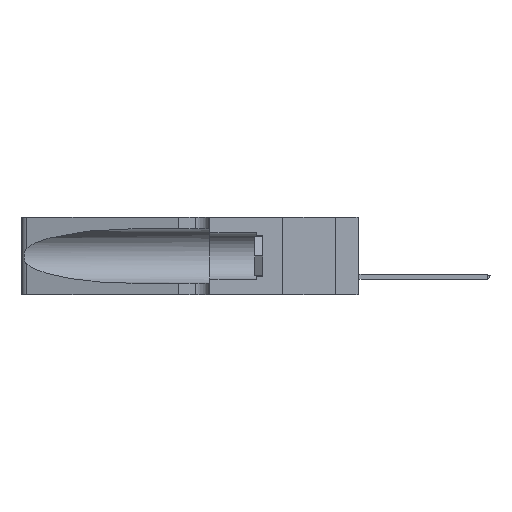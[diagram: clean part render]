
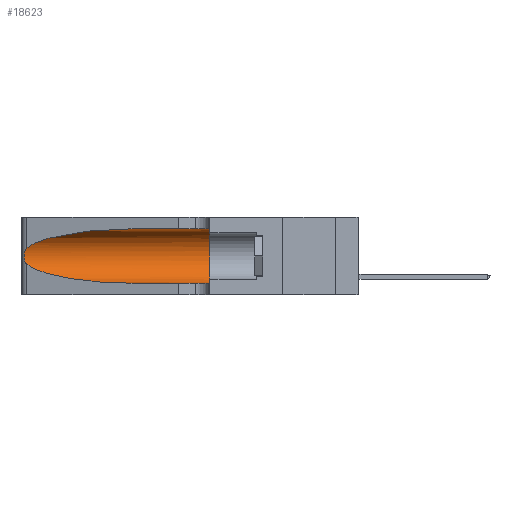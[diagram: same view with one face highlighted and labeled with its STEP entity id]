
A CAD part, left-side view. The second image highlights one B-rep face of the part: STEP entity #18623.
In plain terms, the highlighted cylindrical face has radius 3.308 mm (diameter 6.617 mm), a partial arc.
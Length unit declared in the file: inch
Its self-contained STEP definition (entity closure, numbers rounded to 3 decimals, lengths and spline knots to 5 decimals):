
#246 = VECTOR ( 'NONE', #25116, 39.37008 ) ;
#1058 = EDGE_CURVE ( 'NONE', #35417, #11786, #7215, .T. ) ;
#1437 = CARTESIAN_POINT ( 'NONE',  ( 0.26017, 1.23833, 0.17102 ) ) ;
#1632 = CARTESIAN_POINT ( 'NONE',  ( 0.1305, 1.61858, 0.185 ) ) ;
#3927 = CARTESIAN_POINT ( 'NONE',  ( 0.25487, 1.22718, 0.22369 ) ) ;
#4509 = DIRECTION ( 'NONE',  ( 0., -1., 0. ) ) ;
#4689 = CARTESIAN_POINT ( 'NONE',  ( 0.25555, 1.22994, 0.2215 ) ) ;
#4696 = CARTESIAN_POINT ( 'NONE',  ( 0.1305, 0.72297, 0.05475 ) ) ;
#4701 = CARTESIAN_POINT ( 'NONE',  ( 0.26018, 1.23835, 0.19895 ) ) ;
#5190 = DIRECTION ( 'NONE',  ( 0., 0., 1. ) ) ;
#5891 = ORIENTED_EDGE ( 'NONE', *, *, #9182, .T. ) ;
#6730 = CARTESIAN_POINT ( 'NONE',  ( 0.1305, 1.61858, 0.05475 ) ) ;
#7215 = CIRCLE ( 'NONE', #11530, 0.13025 ) ;
#8630 = AXIS2_PLACEMENT_3D ( 'NONE', #1632, #4509, #35296 ) ;
#8741 = CARTESIAN_POINT ( 'NONE',  ( 0.25787, 1.23484, 0.2124 ) ) ;
#9182 = EDGE_CURVE ( 'NONE', #12603, #26871, #22995, .T. ) ;
#10399 = ORIENTED_EDGE ( 'NONE', *, *, #24437, .F. ) ;
#10614 = CARTESIAN_POINT ( 'NONE',  ( 0.26075, 1.23896, 0.178 ) ) ;
#10651 = EDGE_CURVE ( 'NONE', #34336, #12603, #16984, .T. ) ;
#11083 = CARTESIAN_POINT ( 'NONE',  ( 0.1305, 0.35, 0.05475 ) ) ;
#11516 = CARTESIAN_POINT ( 'NONE',  ( 0.1305, 0.72297, 0.31525 ) ) ;
#11530 = AXIS2_PLACEMENT_3D ( 'NONE', #23554, #29482, #5190 ) ;
#11786 = VERTEX_POINT ( 'NONE', #11083 ) ;
#12603 = VERTEX_POINT ( 'NONE', #26114 ) ;
#14416 = EDGE_LOOP ( 'NONE', ( #18194, #29007, #5891, #35725, #33383, #10399 ) ) ;
#16322 = CARTESIAN_POINT ( 'NONE',  ( 0.1305, 0.72297, 0.31525 ) ) ;
#16454 = CARTESIAN_POINT ( 'NONE',  ( 0.2373, 1.15595, 0.08982 ) ) ;
#16758 = EDGE_CURVE ( 'NONE', #26871, #11786, #29547, .T. ) ;
#16972 = CARTESIAN_POINT ( 'NONE',  ( 0.25789, 1.23486, 0.15765 ) ) ;
#16984 = B_SPLINE_CURVE_WITH_KNOTS ( 'NONE', 3,
 ( #35860, #4689, #36316, #8741, #28080, #4701, #38329, #10614, #1437, #35642, #16972, #17103, #23370, #35098 ),
 .UNSPECIFIED., .F., .F.,
 ( 4, 2, 2, 2, 2, 2, 4 ),
 ( 0., 0.00027, 0.00053, 0.00107, 0.0016, 0.00187, 0.00214 ),
 .UNSPECIFIED. ) ;
#17103 = CARTESIAN_POINT ( 'NONE',  ( 0.25639, 1.23186, 0.15144 ) ) ;
#18045 = LINE ( 'NONE', #27467, #34010 ) ;
#18194 = ORIENTED_EDGE ( 'NONE', *, *, #30231, .T. ) ;
#18623 = ADVANCED_FACE ( 'NONE', ( #35146 ), #33213, .F. ) ;
#19522 = VERTEX_POINT ( 'NONE', #11516 ) ;
#19882 = CARTESIAN_POINT ( 'NONE',  ( 0.1305, 0.72297, 0.05475 ) ) ;
#20011 = CARTESIAN_POINT ( 'NONE',  ( 0.18966, 0.96281, 0.31525 ) ) ;
#22889 = CARTESIAN_POINT ( 'NONE',  ( 0.1305, 0.35, 0.31525 ) ) ;
#22995 =( BOUNDED_CURVE ( )  B_SPLINE_CURVE ( 3, ( #32276, #16454, #32133, #19882 ),
 .UNSPECIFIED., .F., .T. ) 
 B_SPLINE_CURVE_WITH_KNOTS ( ( 4, 4 ),
 ( 3.44316, 4.71239 ),
 .UNSPECIFIED. ) 
 CURVE ( )  GEOMETRIC_REPRESENTATION_ITEM ( )  RATIONAL_B_SPLINE_CURVE ( ( 1., 0.87, 0.87, 1. ) ) 
 REPRESENTATION_ITEM ( '' )  );
#23370 = CARTESIAN_POINT ( 'NONE',  ( 0.25555, 1.22993, 0.14849 ) ) ;
#23497 =( BOUNDED_CURVE ( )  B_SPLINE_CURVE ( 3, ( #16322, #20011, #25699, #3927 ),
 .UNSPECIFIED., .F., .T. ) 
 B_SPLINE_CURVE_WITH_KNOTS ( ( 4, 4 ),
 ( 1.5708, 2.84003 ),
 .UNSPECIFIED. ) 
 CURVE ( )  GEOMETRIC_REPRESENTATION_ITEM ( )  RATIONAL_B_SPLINE_CURVE ( ( 1., 0.87, 0.87, 1. ) ) 
 REPRESENTATION_ITEM ( '' )  );
#23554 = CARTESIAN_POINT ( 'NONE',  ( 0.1305, 0.35, 0.185 ) ) ;
#24437 = EDGE_CURVE ( 'NONE', #19522, #35417, #18045, .T. ) ;
#25116 = DIRECTION ( 'NONE',  ( 0., -1., 0. ) ) ;
#25699 = CARTESIAN_POINT ( 'NONE',  ( 0.2373, 1.15595, 0.28018 ) ) ;
#26114 = CARTESIAN_POINT ( 'NONE',  ( 0.25487, 1.22718, 0.14631 ) ) ;
#26871 = VERTEX_POINT ( 'NONE', #4696 ) ;
#27467 = CARTESIAN_POINT ( 'NONE',  ( 0.1305, 1.61858, 0.31525 ) ) ;
#28080 = CARTESIAN_POINT ( 'NONE',  ( 0.25854, 1.2359, 0.20912 ) ) ;
#29007 = ORIENTED_EDGE ( 'NONE', *, *, #10651, .T. ) ;
#29482 = DIRECTION ( 'NONE',  ( 0., 1., 0. ) ) ;
#29547 = LINE ( 'NONE', #6730, #246 ) ;
#30231 = EDGE_CURVE ( 'NONE', #19522, #34336, #23497, .T. ) ;
#32133 = CARTESIAN_POINT ( 'NONE',  ( 0.18966, 0.96281, 0.05475 ) ) ;
#32276 = CARTESIAN_POINT ( 'NONE',  ( 0.25487, 1.22718, 0.14631 ) ) ;
#33213 = CYLINDRICAL_SURFACE ( 'NONE', #8630, 0.13025 ) ;
#33383 = ORIENTED_EDGE ( 'NONE', *, *, #1058, .F. ) ;
#33535 = DIRECTION ( 'NONE',  ( 0., -1., 0. ) ) ;
#33917 = CARTESIAN_POINT ( 'NONE',  ( 0.25487, 1.22718, 0.22369 ) ) ;
#34010 = VECTOR ( 'NONE', #33535, 39.37008 ) ;
#34336 = VERTEX_POINT ( 'NONE', #33917 ) ;
#35098 = CARTESIAN_POINT ( 'NONE',  ( 0.25487, 1.22718, 0.14631 ) ) ;
#35146 = FACE_OUTER_BOUND ( 'NONE', #14416, .T. ) ;
#35296 = DIRECTION ( 'NONE',  ( 0., 0., -1. ) ) ;
#35417 = VERTEX_POINT ( 'NONE', #22889 ) ;
#35642 = CARTESIAN_POINT ( 'NONE',  ( 0.25856, 1.23593, 0.16098 ) ) ;
#35725 = ORIENTED_EDGE ( 'NONE', *, *, #16758, .T. ) ;
#35860 = CARTESIAN_POINT ( 'NONE',  ( 0.25487, 1.22718, 0.22369 ) ) ;
#36316 = CARTESIAN_POINT ( 'NONE',  ( 0.25639, 1.23184, 0.21858 ) ) ;
#38329 = CARTESIAN_POINT ( 'NONE',  ( 0.26075, 1.23896, 0.19203 ) ) ;
